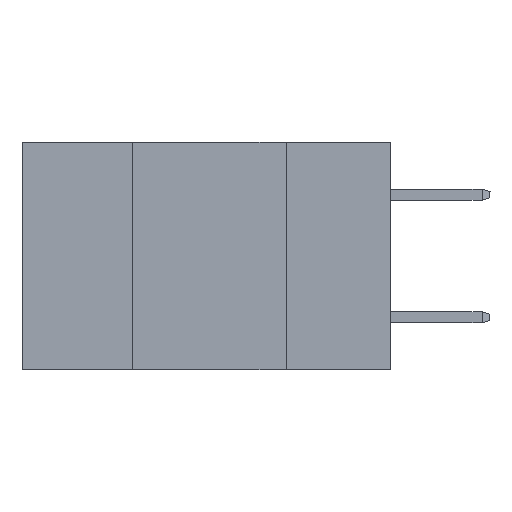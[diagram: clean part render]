
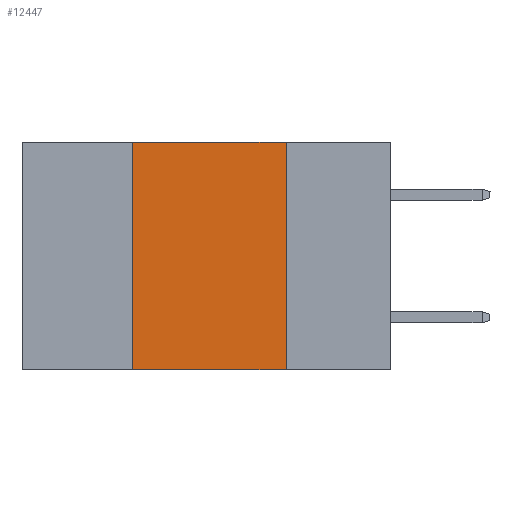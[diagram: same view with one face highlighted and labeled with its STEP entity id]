
A CAD part, left-side view. The second image highlights one B-rep face of the part: STEP entity #12447.
In plain terms, the highlighted planar face has unit normal (-1, 0, 0).
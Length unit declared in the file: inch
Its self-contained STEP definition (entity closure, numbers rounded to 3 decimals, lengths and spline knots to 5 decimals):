
#643 = CARTESIAN_POINT ( 'NONE',  ( 0., 0.6, 0. ) ) ;
#817 = CARTESIAN_POINT ( 'NONE',  ( 0., 0.17, 0. ) ) ;
#984 = CARTESIAN_POINT ( 'NONE',  ( 0., 0.17, -0.37 ) ) ;
#1999 = DIRECTION ( 'NONE',  ( 0., 0., -1. ) ) ;
#2632 = DIRECTION ( 'NONE',  ( 1., 0., 0. ) ) ;
#3768 = VERTEX_POINT ( 'NONE', #14134 ) ;
#3851 = LINE ( 'NONE', #5180, #9655 ) ;
#4002 = LINE ( 'NONE', #13104, #6751 ) ;
#4049 = CARTESIAN_POINT ( 'NONE',  ( 0., 0.42, 0. ) ) ;
#4582 = EDGE_CURVE ( 'NONE', #3768, #4935, #3851, .T. ) ;
#4605 = VECTOR ( 'NONE', #8884, 39.37008 ) ;
#4935 = VERTEX_POINT ( 'NONE', #984 ) ;
#5180 = CARTESIAN_POINT ( 'NONE',  ( 0., 0.6, -0.37 ) ) ;
#5277 = DIRECTION ( 'NONE',  ( 0., -1., 0. ) ) ;
#5333 = VERTEX_POINT ( 'NONE', #9709 ) ;
#5437 = VERTEX_POINT ( 'NONE', #4049 ) ;
#5865 = EDGE_LOOP ( 'NONE', ( #10372, #10398, #10523, #10612 ) ) ;
#6164 = CARTESIAN_POINT ( 'NONE',  ( 0., 0.6, 0. ) ) ;
#6751 = VECTOR ( 'NONE', #8702, 39.37008 ) ;
#7215 = EDGE_CURVE ( 'NONE', #5333, #4935, #12902, .T. ) ;
#8702 = DIRECTION ( 'NONE',  ( 0., 0., 1. ) ) ;
#8884 = DIRECTION ( 'NONE',  ( 0., -1., 0. ) ) ;
#9637 = PLANE ( 'NONE',  #12254 ) ;
#9655 = VECTOR ( 'NONE', #5277, 39.37008 ) ;
#9709 = CARTESIAN_POINT ( 'NONE',  ( 0., 0.17, 0. ) ) ;
#9970 = VECTOR ( 'NONE', #1999, 39.37008 ) ;
#10372 = ORIENTED_EDGE ( 'NONE', *, *, #7215, .F. ) ;
#10398 = ORIENTED_EDGE ( 'NONE', *, *, #11166, .F. ) ;
#10523 = ORIENTED_EDGE ( 'NONE', *, *, #13502, .F. ) ;
#10612 = ORIENTED_EDGE ( 'NONE', *, *, #4582, .T. ) ;
#10767 = DIRECTION ( 'NONE',  ( 0., 0., -1. ) ) ;
#11166 = EDGE_CURVE ( 'NONE', #5437, #5333, #13644, .T. ) ;
#12254 = AXIS2_PLACEMENT_3D ( 'NONE', #6164, #2632, #10767 ) ;
#12447 = ADVANCED_FACE ( 'NONE', ( #14704 ), #9637, .F. ) ;
#12902 = LINE ( 'NONE', #817, #9970 ) ;
#13104 = CARTESIAN_POINT ( 'NONE',  ( 0., 0.42, 0. ) ) ;
#13502 = EDGE_CURVE ( 'NONE', #3768, #5437, #4002, .T. ) ;
#13644 = LINE ( 'NONE', #643, #4605 ) ;
#14134 = CARTESIAN_POINT ( 'NONE',  ( 0., 0.42, -0.37 ) ) ;
#14704 = FACE_OUTER_BOUND ( 'NONE', #5865, .T. ) ;
